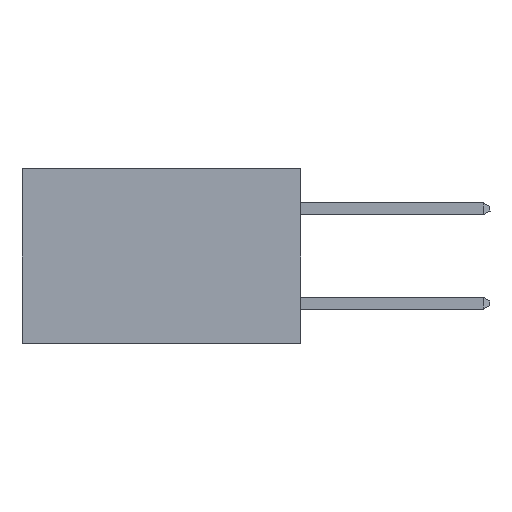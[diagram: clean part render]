
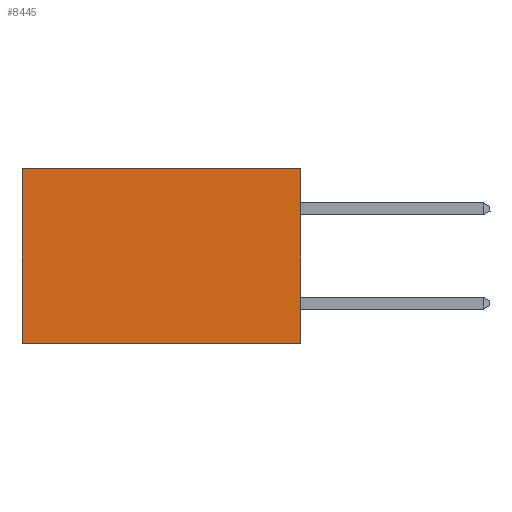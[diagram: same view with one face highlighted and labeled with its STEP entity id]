
A CAD part, left-side view. The second image highlights one B-rep face of the part: STEP entity #8445.
In plain terms, the highlighted planar face has unit normal (-1, 0, 0).
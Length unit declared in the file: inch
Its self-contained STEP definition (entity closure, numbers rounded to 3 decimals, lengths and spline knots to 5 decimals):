
#833 = VECTOR ( 'NONE', #28243, 39.37008 ) ;
#2340 = CARTESIAN_POINT ( 'NONE',  ( 0.277, 0., 0. ) ) ;
#3355 = CARTESIAN_POINT ( 'NONE',  ( 0.277, 0., -0.37 ) ) ;
#3492 = PLANE ( 'NONE',  #28956 ) ;
#4235 = LINE ( 'NONE', #30879, #24206 ) ;
#8445 = ADVANCED_FACE ( 'NONE', ( #30351 ), #3492, .F. ) ;
#11391 = VERTEX_POINT ( 'NONE', #20010 ) ;
#12981 = EDGE_CURVE ( 'NONE', #27980, #18034, #4235, .T. ) ;
#13499 = CARTESIAN_POINT ( 'NONE',  ( 0.277, 0.59, -0.37 ) ) ;
#13522 = DIRECTION ( 'NONE',  ( 0., 0., -1. ) ) ;
#13641 = ORIENTED_EDGE ( 'NONE', *, *, #28363, .T. ) ;
#15543 = CARTESIAN_POINT ( 'NONE',  ( 0.277, 0.59, 0. ) ) ;
#16208 = DIRECTION ( 'NONE',  ( 0., 1., 0. ) ) ;
#18034 = VERTEX_POINT ( 'NONE', #29310 ) ;
#18344 = ORIENTED_EDGE ( 'NONE', *, *, #22734, .T. ) ;
#18538 = CARTESIAN_POINT ( 'NONE',  ( 0.277, 0., -0.37 ) ) ;
#19062 = VERTEX_POINT ( 'NONE', #15543 ) ;
#20010 = CARTESIAN_POINT ( 'NONE',  ( 0.277, 0.59, -0.37 ) ) ;
#20603 = VECTOR ( 'NONE', #16208, 39.37008 ) ;
#22734 = EDGE_CURVE ( 'NONE', #19062, #11391, #30548, .T. ) ;
#23707 = EDGE_CURVE ( 'NONE', #18034, #11391, #27422, .T. ) ;
#24206 = VECTOR ( 'NONE', #25953, 39.37008 ) ;
#24782 = VECTOR ( 'NONE', #30928, 39.37008 ) ;
#25953 = DIRECTION ( 'NONE',  ( 0., 0., -1. ) ) ;
#26130 = ORIENTED_EDGE ( 'NONE', *, *, #12981, .F. ) ;
#26165 = CARTESIAN_POINT ( 'NONE',  ( 0.277, 0., 0. ) ) ;
#27168 = LINE ( 'NONE', #26165, #20603 ) ;
#27422 = LINE ( 'NONE', #3355, #833 ) ;
#27980 = VERTEX_POINT ( 'NONE', #2340 ) ;
#28243 = DIRECTION ( 'NONE',  ( 0., 1., 0. ) ) ;
#28363 = EDGE_CURVE ( 'NONE', #27980, #19062, #27168, .T. ) ;
#28488 = DIRECTION ( 'NONE',  ( 1., 0., 0. ) ) ;
#28956 = AXIS2_PLACEMENT_3D ( 'NONE', #18538, #28488, #13522 ) ;
#29310 = CARTESIAN_POINT ( 'NONE',  ( 0.277, 0., -0.37 ) ) ;
#30351 = FACE_OUTER_BOUND ( 'NONE', #30529, .T. ) ;
#30529 = EDGE_LOOP ( 'NONE', ( #18344, #31162, #26130, #13641 ) ) ;
#30548 = LINE ( 'NONE', #13499, #24782 ) ;
#30879 = CARTESIAN_POINT ( 'NONE',  ( 0.277, 0., -0.37 ) ) ;
#30928 = DIRECTION ( 'NONE',  ( 0., 0., -1. ) ) ;
#31162 = ORIENTED_EDGE ( 'NONE', *, *, #23707, .F. ) ;
